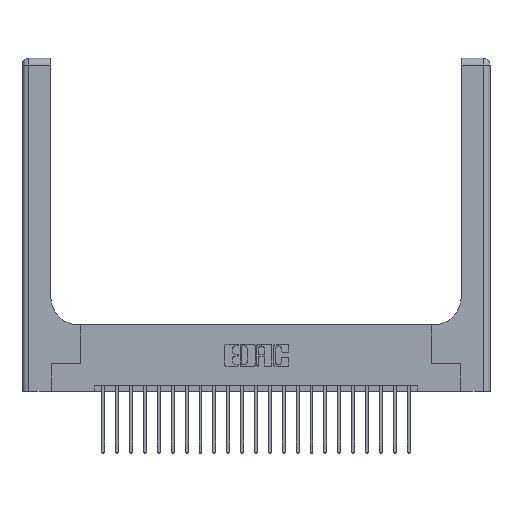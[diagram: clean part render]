
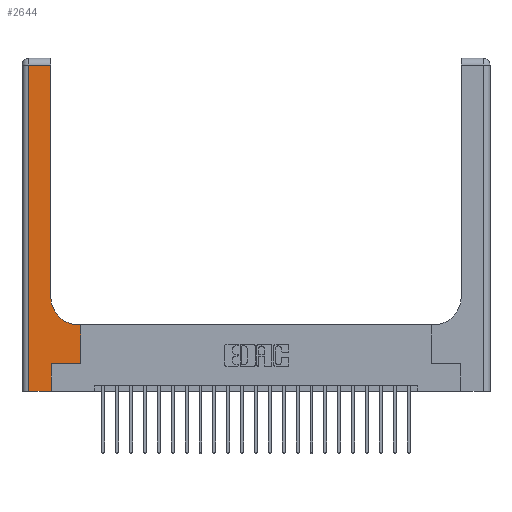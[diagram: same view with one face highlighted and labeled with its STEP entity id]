
A CAD part, top view. The second image highlights one B-rep face of the part: STEP entity #2644.
In plain terms, the highlighted planar face has unit normal (0, 0, 1).
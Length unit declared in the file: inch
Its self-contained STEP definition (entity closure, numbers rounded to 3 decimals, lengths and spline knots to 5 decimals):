
#1044 = ORIENTED_EDGE ( 'NONE', *, *, #22180, .T. ) ;
#1315 = VECTOR ( 'NONE', #4522, 39.37008 ) ;
#1436 = DIRECTION ( 'NONE',  ( 1., 0., 0. ) ) ;
#1536 = VERTEX_POINT ( 'NONE', #20071 ) ;
#1958 = CARTESIAN_POINT ( 'NONE',  ( 0.26, 3., 0.37 ) ) ;
#2189 = FACE_OUTER_BOUND ( 'NONE', #21993, .T. ) ;
#2644 = ADVANCED_FACE ( 'NONE', ( #2189 ), #20751, .F. ) ;
#2723 = CARTESIAN_POINT ( 'NONE',  ( 0.265, 0., 0.37 ) ) ;
#2742 = ORIENTED_EDGE ( 'NONE', *, *, #22439, .T. ) ;
#2934 = VECTOR ( 'NONE', #20562, 39.37008 ) ;
#2974 = CARTESIAN_POINT ( 'NONE',  ( 0.51, 0.85, 0.37 ) ) ;
#3113 = LINE ( 'NONE', #21981, #12172 ) ;
#3196 = DIRECTION ( 'NONE',  ( 0., 0., -1. ) ) ;
#3355 = DIRECTION ( 'NONE',  ( -1., 0., 0. ) ) ;
#3397 = CARTESIAN_POINT ( 'NONE',  ( 0.528, 0.25, 0.37 ) ) ;
#3460 = LINE ( 'NONE', #11702, #12508 ) ;
#4522 = DIRECTION ( 'NONE',  ( -1., 0., 0. ) ) ;
#4565 = EDGE_CURVE ( 'NONE', #11640, #13762, #3460, .T. ) ;
#5220 = ORIENTED_EDGE ( 'NONE', *, *, #22416, .T. ) ;
#5292 = DIRECTION ( 'NONE',  ( 1., 0., 0. ) ) ;
#5453 = VERTEX_POINT ( 'NONE', #7596 ) ;
#5535 = LINE ( 'NONE', #12129, #9389 ) ;
#5825 = LINE ( 'NONE', #1958, #21245 ) ;
#6252 = CARTESIAN_POINT ( 'NONE',  ( 0.06, 0., 0.37 ) ) ;
#6277 = EDGE_CURVE ( 'NONE', #16146, #18384, #5825, .T. ) ;
#6894 = LINE ( 'NONE', #15293, #17647 ) ;
#7596 = CARTESIAN_POINT ( 'NONE',  ( 0.528, 0.6, 0.37 ) ) ;
#8705 = CARTESIAN_POINT ( 'NONE',  ( 0.265, 0.25, 0.37 ) ) ;
#9389 = VECTOR ( 'NONE', #5292, 39.37008 ) ;
#9418 = CARTESIAN_POINT ( 'NONE',  ( 0., 2.94, 0.37 ) ) ;
#10629 = CARTESIAN_POINT ( 'NONE',  ( 0.26, 0.85, 0.37 ) ) ;
#11223 = VECTOR ( 'NONE', #21716, 39.37008 ) ;
#11640 = VERTEX_POINT ( 'NONE', #16312 ) ;
#11702 = CARTESIAN_POINT ( 'NONE',  ( 0.06, 3., 0.37 ) ) ;
#11827 = EDGE_CURVE ( 'NONE', #5453, #1536, #21659, .T. ) ;
#12006 = CARTESIAN_POINT ( 'NONE',  ( 0., 3., 0.37 ) ) ;
#12129 = CARTESIAN_POINT ( 'NONE',  ( 0.265, 0.25, 0.37 ) ) ;
#12172 = VECTOR ( 'NONE', #22147, 39.37008 ) ;
#12280 = DIRECTION ( 'NONE',  ( 1., 0., 0. ) ) ;
#12408 = VERTEX_POINT ( 'NONE', #8705 ) ;
#12508 = VECTOR ( 'NONE', #18796, 39.37008 ) ;
#13257 = AXIS2_PLACEMENT_3D ( 'NONE', #12006, #19120, #3355 ) ;
#13338 = CARTESIAN_POINT ( 'NONE',  ( 0.26, 2.94, 0.37 ) ) ;
#13762 = VERTEX_POINT ( 'NONE', #6252 ) ;
#13927 = DIRECTION ( 'NONE',  ( 0., 1., 0. ) ) ;
#13986 = ORIENTED_EDGE ( 'NONE', *, *, #14939, .T. ) ;
#13990 = LINE ( 'NONE', #9418, #11223 ) ;
#14178 = LINE ( 'NONE', #2723, #2934 ) ;
#14192 = EDGE_CURVE ( 'NONE', #16064, #12408, #14178, .T. ) ;
#14386 = ORIENTED_EDGE ( 'NONE', *, *, #14192, .T. ) ;
#14547 = ORIENTED_EDGE ( 'NONE', *, *, #11827, .T. ) ;
#14939 = EDGE_CURVE ( 'NONE', #1536, #16146, #21603, .T. ) ;
#15293 = CARTESIAN_POINT ( 'NONE',  ( 0., 0., 0.37 ) ) ;
#15775 = CARTESIAN_POINT ( 'NONE',  ( 0.265, 0., 0.37 ) ) ;
#16057 = AXIS2_PLACEMENT_3D ( 'NONE', #2974, #3196, #1436 ) ;
#16064 = VERTEX_POINT ( 'NONE', #15775 ) ;
#16146 = VERTEX_POINT ( 'NONE', #10629 ) ;
#16312 = CARTESIAN_POINT ( 'NONE',  ( 0.06, 2.94, 0.37 ) ) ;
#17033 = EDGE_CURVE ( 'NONE', #18384, #11640, #13990, .T. ) ;
#17446 = ORIENTED_EDGE ( 'NONE', *, *, #4565, .T. ) ;
#17647 = VECTOR ( 'NONE', #12280, 39.37008 ) ;
#18384 = VERTEX_POINT ( 'NONE', #13338 ) ;
#18796 = DIRECTION ( 'NONE',  ( 0., -1., 0. ) ) ;
#18850 = ORIENTED_EDGE ( 'NONE', *, *, #6277, .T. ) ;
#19035 = ORIENTED_EDGE ( 'NONE', *, *, #17033, .T. ) ;
#19120 = DIRECTION ( 'NONE',  ( 0., 0., -1. ) ) ;
#20071 = CARTESIAN_POINT ( 'NONE',  ( 0.51, 0.6, 0.37 ) ) ;
#20562 = DIRECTION ( 'NONE',  ( 0., 1., 0. ) ) ;
#20751 = PLANE ( 'NONE',  #13257 ) ;
#21245 = VECTOR ( 'NONE', #13927, 39.37008 ) ;
#21603 = CIRCLE ( 'NONE', #16057, 0.25 ) ;
#21659 = LINE ( 'NONE', #22161, #1315 ) ;
#21716 = DIRECTION ( 'NONE',  ( -1., 0., 0. ) ) ;
#21981 = CARTESIAN_POINT ( 'NONE',  ( 0.528, 0.25, 0.37 ) ) ;
#21993 = EDGE_LOOP ( 'NONE', ( #18850, #19035, #17446, #5220, #14386, #2742, #1044, #14547, #13986 ) ) ;
#22147 = DIRECTION ( 'NONE',  ( 0., 1., 0. ) ) ;
#22161 = CARTESIAN_POINT ( 'NONE',  ( 0.26, 0.6, 0.37 ) ) ;
#22180 = EDGE_CURVE ( 'NONE', #22475, #5453, #3113, .T. ) ;
#22416 = EDGE_CURVE ( 'NONE', #13762, #16064, #6894, .T. ) ;
#22439 = EDGE_CURVE ( 'NONE', #12408, #22475, #5535, .T. ) ;
#22475 = VERTEX_POINT ( 'NONE', #3397 ) ;
